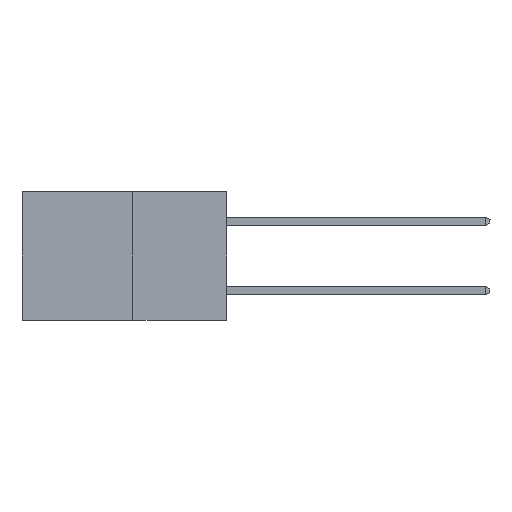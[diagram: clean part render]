
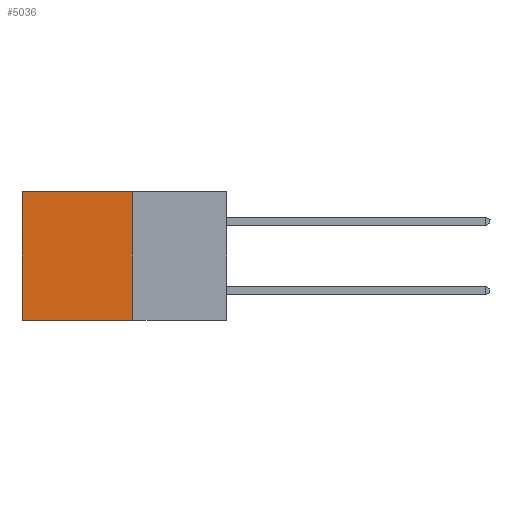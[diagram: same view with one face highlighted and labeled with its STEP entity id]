
A CAD part, left-side view. The second image highlights one B-rep face of the part: STEP entity #5036.
In plain terms, the highlighted planar face has unit normal (-1, 0, 0).
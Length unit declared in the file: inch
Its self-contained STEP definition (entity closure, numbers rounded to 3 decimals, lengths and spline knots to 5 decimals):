
#140 = CARTESIAN_POINT ( 'NONE',  ( 0.277, 0.27, -0.37 ) ) ;
#999 = VERTEX_POINT ( 'NONE', #8097 ) ;
#1193 = VERTEX_POINT ( 'NONE', #3421 ) ;
#1338 = EDGE_LOOP ( 'NONE', ( #4873, #7808, #11476, #3002 ) ) ;
#1375 = VECTOR ( 'NONE', #5730, 39.37008 ) ;
#2267 = DIRECTION ( 'NONE',  ( 0., 0., -1. ) ) ;
#2285 = DIRECTION ( 'NONE',  ( 1., 0., 0. ) ) ;
#2640 = PLANE ( 'NONE',  #4931 ) ;
#2892 = CARTESIAN_POINT ( 'NONE',  ( 0.277, 0.27, -0.37 ) ) ;
#3002 = ORIENTED_EDGE ( 'NONE', *, *, #8642, .T. ) ;
#3005 = VECTOR ( 'NONE', #4182, 39.37008 ) ;
#3421 = CARTESIAN_POINT ( 'NONE',  ( 0.277, 0.59, -0.37 ) ) ;
#3561 = CARTESIAN_POINT ( 'NONE',  ( 0.277, 0.27, 0. ) ) ;
#4005 = VECTOR ( 'NONE', #8302, 39.37008 ) ;
#4182 = DIRECTION ( 'NONE',  ( 0., 1., 0. ) ) ;
#4233 = EDGE_CURVE ( 'NONE', #13935, #1193, #10429, .T. ) ;
#4266 = LINE ( 'NONE', #3561, #1375 ) ;
#4401 = EDGE_CURVE ( 'NONE', #6309, #13935, #13860, .T. ) ;
#4862 = CARTESIAN_POINT ( 'NONE',  ( 0.277, 0.27, -0.37 ) ) ;
#4873 = ORIENTED_EDGE ( 'NONE', *, *, #13260, .T. ) ;
#4931 = AXIS2_PLACEMENT_3D ( 'NONE', #2892, #2285, #2267 ) ;
#5036 = ADVANCED_FACE ( 'NONE', ( #8815 ), #2640, .F. ) ;
#5045 = VECTOR ( 'NONE', #11701, 39.37008 ) ;
#5730 = DIRECTION ( 'NONE',  ( 0., 1., 0. ) ) ;
#6309 = VERTEX_POINT ( 'NONE', #11393 ) ;
#7808 = ORIENTED_EDGE ( 'NONE', *, *, #4233, .F. ) ;
#8097 = CARTESIAN_POINT ( 'NONE',  ( 0.277, 0.59, 0. ) ) ;
#8302 = DIRECTION ( 'NONE',  ( 0., 0., -1. ) ) ;
#8642 = EDGE_CURVE ( 'NONE', #6309, #999, #4266, .T. ) ;
#8815 = FACE_OUTER_BOUND ( 'NONE', #1338, .T. ) ;
#10429 = LINE ( 'NONE', #140, #3005 ) ;
#11393 = CARTESIAN_POINT ( 'NONE',  ( 0.277, 0.27, 0. ) ) ;
#11476 = ORIENTED_EDGE ( 'NONE', *, *, #4401, .F. ) ;
#11701 = DIRECTION ( 'NONE',  ( 0., 0., -1. ) ) ;
#11869 = CARTESIAN_POINT ( 'NONE',  ( 0.277, 0.27, -0.37 ) ) ;
#12808 = LINE ( 'NONE', #13804, #4005 ) ;
#13260 = EDGE_CURVE ( 'NONE', #999, #1193, #12808, .T. ) ;
#13804 = CARTESIAN_POINT ( 'NONE',  ( 0.277, 0.59, -0.37 ) ) ;
#13860 = LINE ( 'NONE', #11869, #5045 ) ;
#13935 = VERTEX_POINT ( 'NONE', #4862 ) ;
